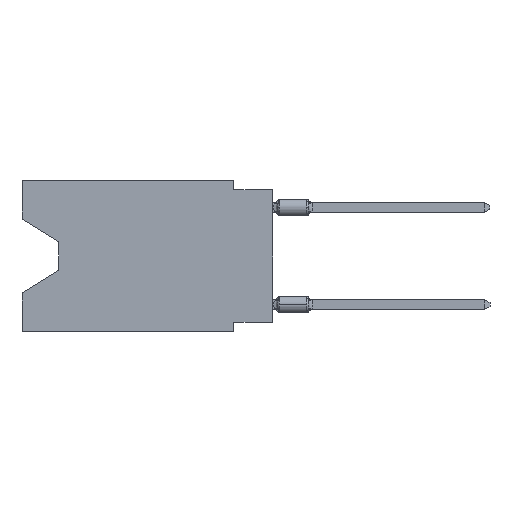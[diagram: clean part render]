
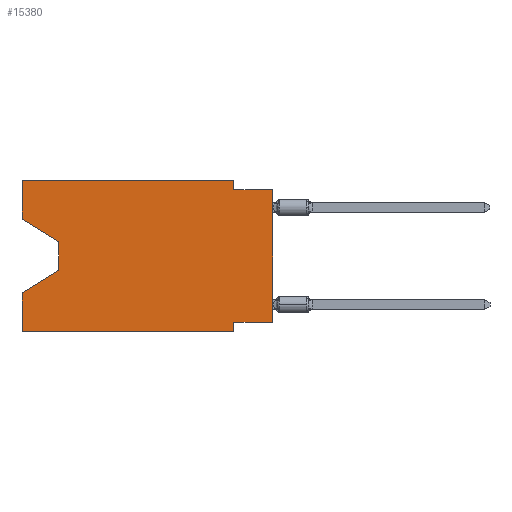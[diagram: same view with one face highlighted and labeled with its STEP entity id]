
A CAD part, left-side view. The second image highlights one B-rep face of the part: STEP entity #15380.
In plain terms, the highlighted planar face has unit normal (-1, 0, 0).
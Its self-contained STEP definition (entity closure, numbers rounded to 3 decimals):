
#172 = LINE ( 'NONE', #25567, #13074 ) ;
#354 = EDGE_CURVE ( 'NONE', #18465, #5645, #14900, .T. ) ;
#882 = ORIENTED_EDGE ( 'NONE', *, *, #12726, .F. ) ;
#1249 = DIRECTION ( 'NONE',  ( 0., 0., -1. ) ) ;
#1364 = CARTESIAN_POINT ( 'NONE',  ( 0., 2.54, -9.906 ) ) ;
#1385 = CARTESIAN_POINT ( 'NONE',  ( 0., 16.383, -9.906 ) ) ;
#1443 = CARTESIAN_POINT ( 'NONE',  ( 0., 16.383, 0. ) ) ;
#2062 = VERTEX_POINT ( 'NONE', #25077 ) ;
#2340 = CARTESIAN_POINT ( 'NONE',  ( 0., 16.383, -2.546 ) ) ;
#2687 = PLANE ( 'NONE',  #8680 ) ;
#3082 = VERTEX_POINT ( 'NONE', #21558 ) ;
#3781 = CARTESIAN_POINT ( 'NONE',  ( 0., 16.383, 0. ) ) ;
#3889 = VECTOR ( 'NONE', #24821, 1000. ) ;
#4191 = DIRECTION ( 'NONE',  ( 0., 0., 1. ) ) ;
#4692 = DIRECTION ( 'NONE',  ( 0., 0.855, -0.519 ) ) ;
#4857 = VECTOR ( 'NONE', #11108, 1000. ) ;
#5116 = VERTEX_POINT ( 'NONE', #7013 ) ;
#5305 = DIRECTION ( 'NONE',  ( 0., 0., -1. ) ) ;
#5342 = DIRECTION ( 'NONE',  ( 0., -1., 0. ) ) ;
#5472 = VERTEX_POINT ( 'NONE', #17428 ) ;
#5645 = VERTEX_POINT ( 'NONE', #18064 ) ;
#6621 = DIRECTION ( 'NONE',  ( 0., -0.855, -0.519 ) ) ;
#7013 = CARTESIAN_POINT ( 'NONE',  ( 0., 2.54, -9.271 ) ) ;
#7093 = FACE_OUTER_BOUND ( 'NONE', #20366, .T. ) ;
#7749 = ORIENTED_EDGE ( 'NONE', *, *, #11563, .T. ) ;
#7990 = CARTESIAN_POINT ( 'NONE',  ( 0., 0., -9.271 ) ) ;
#8012 = CARTESIAN_POINT ( 'NONE',  ( 0., 0., 0. ) ) ;
#8650 = VECTOR ( 'NONE', #21018, 1000. ) ;
#8680 = AXIS2_PLACEMENT_3D ( 'NONE', #18504, #18737, #1249 ) ;
#8932 = LINE ( 'NONE', #1385, #3889 ) ;
#9072 = ORIENTED_EDGE ( 'NONE', *, *, #20974, .T. ) ;
#9132 = VERTEX_POINT ( 'NONE', #18185 ) ;
#9194 = LINE ( 'NONE', #12622, #18134 ) ;
#9869 = EDGE_CURVE ( 'NONE', #2062, #23505, #23164, .T. ) ;
#9941 = CARTESIAN_POINT ( 'NONE',  ( 0., 2.54, -9.906 ) ) ;
#10794 = VERTEX_POINT ( 'NONE', #16669 ) ;
#10884 = EDGE_CURVE ( 'NONE', #5116, #14297, #19126, .T. ) ;
#10945 = VECTOR ( 'NONE', #11765, 1000. ) ;
#11059 = ORIENTED_EDGE ( 'NONE', *, *, #354, .T. ) ;
#11108 = DIRECTION ( 'NONE',  ( 0., 0., -1. ) ) ;
#11149 = CARTESIAN_POINT ( 'NONE',  ( 0., 0., -0.635 ) ) ;
#11438 = VECTOR ( 'NONE', #5305, 1000. ) ;
#11454 = VECTOR ( 'NONE', #19042, 1000. ) ;
#11563 = EDGE_CURVE ( 'NONE', #5645, #3082, #9194, .T. ) ;
#11765 = DIRECTION ( 'NONE',  ( 0., 1., 0. ) ) ;
#11772 = CARTESIAN_POINT ( 'NONE',  ( 0., 0., -0.635 ) ) ;
#12290 = CARTESIAN_POINT ( 'NONE',  ( 0., 16.383, -9.906 ) ) ;
#12622 = CARTESIAN_POINT ( 'NONE',  ( 0., 13.97, -5.893 ) ) ;
#12642 = ORIENTED_EDGE ( 'NONE', *, *, #18380, .F. ) ;
#12726 = EDGE_CURVE ( 'NONE', #10794, #5472, #25000, .T. ) ;
#12946 = VECTOR ( 'NONE', #5342, 1000. ) ;
#13074 = VECTOR ( 'NONE', #4191, 1000. ) ;
#13182 = LINE ( 'NONE', #22480, #13818 ) ;
#13656 = LINE ( 'NONE', #3781, #12946 ) ;
#13818 = VECTOR ( 'NONE', #14860, 1000. ) ;
#14297 = VERTEX_POINT ( 'NONE', #9941 ) ;
#14789 = EDGE_CURVE ( 'NONE', #10794, #18465, #16193, .T. ) ;
#14860 = DIRECTION ( 'NONE',  ( 0., 0., -1. ) ) ;
#14900 = LINE ( 'NONE', #23033, #11438 ) ;
#15380 = ADVANCED_FACE ( 'NONE', ( #7093 ), #2687, .F. ) ;
#15872 = ORIENTED_EDGE ( 'NONE', *, *, #25133, .F. ) ;
#16193 = LINE ( 'NONE', #2340, #24749 ) ;
#16669 = CARTESIAN_POINT ( 'NONE',  ( 0., 16.383, -2.546 ) ) ;
#16857 = VERTEX_POINT ( 'NONE', #20924 ) ;
#17426 = EDGE_CURVE ( 'NONE', #5472, #9132, #13656, .T. ) ;
#17428 = CARTESIAN_POINT ( 'NONE',  ( 0., 16.383, 0. ) ) ;
#17510 = ORIENTED_EDGE ( 'NONE', *, *, #17426, .F. ) ;
#17581 = LINE ( 'NONE', #7990, #10945 ) ;
#18064 = CARTESIAN_POINT ( 'NONE',  ( 0., 13.97, -5.893 ) ) ;
#18134 = VECTOR ( 'NONE', #4692, 1000. ) ;
#18185 = CARTESIAN_POINT ( 'NONE',  ( 0., 2.54, 0. ) ) ;
#18380 = EDGE_CURVE ( 'NONE', #9132, #2062, #13182, .T. ) ;
#18465 = VERTEX_POINT ( 'NONE', #19115 ) ;
#18504 = CARTESIAN_POINT ( 'NONE',  ( 0., 16.383, 0. ) ) ;
#18737 = DIRECTION ( 'NONE',  ( 1., 0., 0. ) ) ;
#19042 = DIRECTION ( 'NONE',  ( 0., -1., 0. ) ) ;
#19115 = CARTESIAN_POINT ( 'NONE',  ( 0., 13.97, -4.013 ) ) ;
#19126 = LINE ( 'NONE', #1364, #4857 ) ;
#19583 = VECTOR ( 'NONE', #23797, 1000. ) ;
#20366 = EDGE_LOOP ( 'NONE', ( #24799, #11059, #7749, #15872, #21126, #20424, #22212, #9072, #21263, #12642, #17510, #882 ) ) ;
#20424 = ORIENTED_EDGE ( 'NONE', *, *, #10884, .F. ) ;
#20924 = CARTESIAN_POINT ( 'NONE',  ( 0., 0., -9.271 ) ) ;
#20974 = EDGE_CURVE ( 'NONE', #16857, #23505, #22338, .T. ) ;
#21018 = DIRECTION ( 'NONE',  ( 0., 0., 1. ) ) ;
#21126 = ORIENTED_EDGE ( 'NONE', *, *, #21771, .T. ) ;
#21263 = ORIENTED_EDGE ( 'NONE', *, *, #9869, .F. ) ;
#21558 = CARTESIAN_POINT ( 'NONE',  ( 0., 16.383, -7.36 ) ) ;
#21771 = EDGE_CURVE ( 'NONE', #24887, #14297, #8932, .T. ) ;
#22212 = ORIENTED_EDGE ( 'NONE', *, *, #22269, .F. ) ;
#22269 = EDGE_CURVE ( 'NONE', #16857, #5116, #17581, .T. ) ;
#22338 = LINE ( 'NONE', #8012, #19583 ) ;
#22480 = CARTESIAN_POINT ( 'NONE',  ( 0., 2.54, 0. ) ) ;
#23033 = CARTESIAN_POINT ( 'NONE',  ( 0., 13.97, -4.013 ) ) ;
#23164 = LINE ( 'NONE', #11149, #11454 ) ;
#23505 = VERTEX_POINT ( 'NONE', #11772 ) ;
#23797 = DIRECTION ( 'NONE',  ( 0., 0., 1. ) ) ;
#24749 = VECTOR ( 'NONE', #6621, 1000. ) ;
#24799 = ORIENTED_EDGE ( 'NONE', *, *, #14789, .T. ) ;
#24821 = DIRECTION ( 'NONE',  ( 0., -1., 0. ) ) ;
#24887 = VERTEX_POINT ( 'NONE', #12290 ) ;
#25000 = LINE ( 'NONE', #1443, #8650 ) ;
#25077 = CARTESIAN_POINT ( 'NONE',  ( 0., 2.54, -0.635 ) ) ;
#25133 = EDGE_CURVE ( 'NONE', #24887, #3082, #172, .T. ) ;
#25567 = CARTESIAN_POINT ( 'NONE',  ( 0., 16.383, 0. ) ) ;
